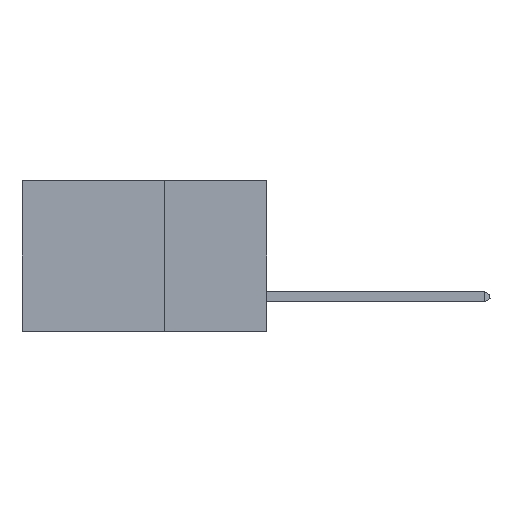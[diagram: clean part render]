
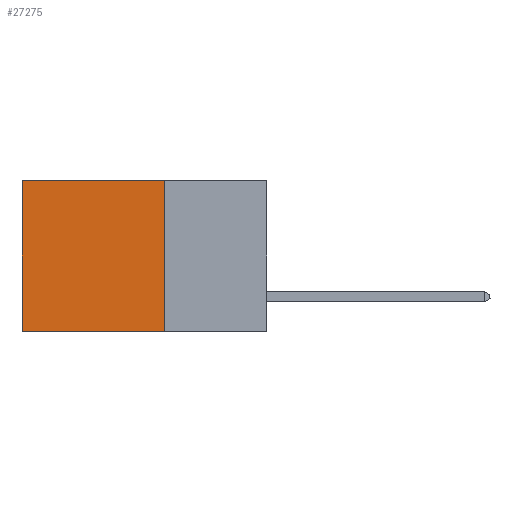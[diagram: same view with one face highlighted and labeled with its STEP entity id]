
A CAD part, left-side view. The second image highlights one B-rep face of the part: STEP entity #27275.
In plain terms, the highlighted planar face has unit normal (-1, 0, 0).
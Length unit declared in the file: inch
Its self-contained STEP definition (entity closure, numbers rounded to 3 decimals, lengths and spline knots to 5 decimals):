
#942 = LINE ( 'NONE', #25463, #27382 ) ;
#1500 = AXIS2_PLACEMENT_3D ( 'NONE', #18363, #2062, #7788 ) ;
#2062 = DIRECTION ( 'NONE',  ( 1., 0., 0. ) ) ;
#2087 = EDGE_CURVE ( 'NONE', #34342, #10367, #23996, .T. ) ;
#2153 = DIRECTION ( 'NONE',  ( 0., 1., 0. ) ) ;
#2274 = CARTESIAN_POINT ( 'NONE',  ( 0.2875, 0.25, -0.37 ) ) ;
#3370 = CARTESIAN_POINT ( 'NONE',  ( 0.2875, 0.25, 0. ) ) ;
#4444 = DIRECTION ( 'NONE',  ( 0., 1., 0. ) ) ;
#6328 = EDGE_CURVE ( 'NONE', #12294, #34342, #28881, .T. ) ;
#7788 = DIRECTION ( 'NONE',  ( 0., 0., -1. ) ) ;
#8207 = VECTOR ( 'NONE', #2153, 39.37008 ) ;
#9239 = CARTESIAN_POINT ( 'NONE',  ( 0.2875, 0.25, -0.37 ) ) ;
#9963 = ORIENTED_EDGE ( 'NONE', *, *, #18250, .T. ) ;
#10367 = VERTEX_POINT ( 'NONE', #25902 ) ;
#12294 = VERTEX_POINT ( 'NONE', #3370 ) ;
#13331 = FACE_OUTER_BOUND ( 'NONE', #21839, .T. ) ;
#13987 = ORIENTED_EDGE ( 'NONE', *, *, #15282, .T. ) ;
#15282 = EDGE_CURVE ( 'NONE', #12294, #24923, #17700, .T. ) ;
#15628 = PLANE ( 'NONE',  #1500 ) ;
#15741 = ORIENTED_EDGE ( 'NONE', *, *, #6328, .F. ) ;
#17446 = DIRECTION ( 'NONE',  ( 0., 0., -1. ) ) ;
#17700 = LINE ( 'NONE', #28887, #24128 ) ;
#18250 = EDGE_CURVE ( 'NONE', #24923, #10367, #942, .T. ) ;
#18363 = CARTESIAN_POINT ( 'NONE',  ( 0.2875, 0.25, 0. ) ) ;
#21067 = CARTESIAN_POINT ( 'NONE',  ( 0.2875, 0.25, 0. ) ) ;
#21839 = EDGE_LOOP ( 'NONE', ( #9963, #30319, #15741, #13987 ) ) ;
#23996 = LINE ( 'NONE', #2274, #8207 ) ;
#24128 = VECTOR ( 'NONE', #4444, 39.37008 ) ;
#24923 = VERTEX_POINT ( 'NONE', #30736 ) ;
#25463 = CARTESIAN_POINT ( 'NONE',  ( 0.2875, 0.6, 0. ) ) ;
#25902 = CARTESIAN_POINT ( 'NONE',  ( 0.2875, 0.6, -0.37 ) ) ;
#26334 = VECTOR ( 'NONE', #26710, 39.37008 ) ;
#26710 = DIRECTION ( 'NONE',  ( 0., 0., -1. ) ) ;
#27275 = ADVANCED_FACE ( 'NONE', ( #13331 ), #15628, .F. ) ;
#27382 = VECTOR ( 'NONE', #17446, 39.37008 ) ;
#28881 = LINE ( 'NONE', #21067, #26334 ) ;
#28887 = CARTESIAN_POINT ( 'NONE',  ( 0.2875, 0.25, 0. ) ) ;
#30319 = ORIENTED_EDGE ( 'NONE', *, *, #2087, .F. ) ;
#30736 = CARTESIAN_POINT ( 'NONE',  ( 0.2875, 0.6, 0. ) ) ;
#34342 = VERTEX_POINT ( 'NONE', #9239 ) ;
